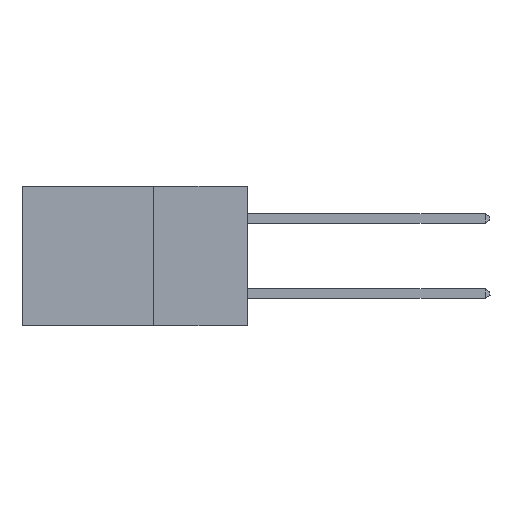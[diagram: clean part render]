
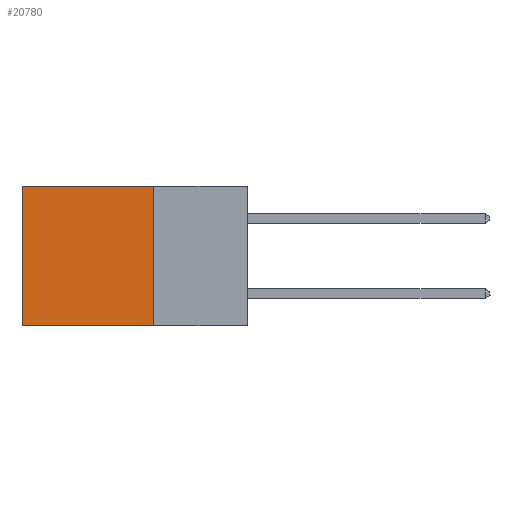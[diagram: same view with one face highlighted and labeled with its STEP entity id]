
A CAD part, left-side view. The second image highlights one B-rep face of the part: STEP entity #20780.
In plain terms, the highlighted planar face has unit normal (-1, 0, 0).
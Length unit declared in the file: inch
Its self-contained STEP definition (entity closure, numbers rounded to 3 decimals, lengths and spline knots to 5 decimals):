
#270 = VECTOR ( 'NONE', #4912, 39.37008 ) ;
#972 = CARTESIAN_POINT ( 'NONE',  ( 0.298, 0.25, 0. ) ) ;
#4577 = LINE ( 'NONE', #8691, #10844 ) ;
#4910 = CARTESIAN_POINT ( 'NONE',  ( 0.298, 0.6, -0.37 ) ) ;
#4912 = DIRECTION ( 'NONE',  ( 0., 0., -1. ) ) ;
#6288 = EDGE_CURVE ( 'NONE', #12097, #23439, #10033, .T. ) ;
#6700 = CARTESIAN_POINT ( 'NONE',  ( 0.298, 0.25, 0. ) ) ;
#6962 = DIRECTION ( 'NONE',  ( 1., 0., 0. ) ) ;
#7075 = PLANE ( 'NONE',  #17705 ) ;
#7313 = EDGE_LOOP ( 'NONE', ( #16508, #26935, #26849, #10260 ) ) ;
#7542 = DIRECTION ( 'NONE',  ( 0., 0., -1. ) ) ;
#7704 = VECTOR ( 'NONE', #7542, 39.37008 ) ;
#7769 = EDGE_CURVE ( 'NONE', #19668, #12097, #17508, .T. ) ;
#8394 = LINE ( 'NONE', #972, #7704 ) ;
#8691 = CARTESIAN_POINT ( 'NONE',  ( 0.298, 0.25, -0.37 ) ) ;
#9128 = CARTESIAN_POINT ( 'NONE',  ( 0.298, 0.6, 0. ) ) ;
#9564 = EDGE_CURVE ( 'NONE', #24120, #23439, #4577, .T. ) ;
#10033 = LINE ( 'NONE', #9128, #270 ) ;
#10260 = ORIENTED_EDGE ( 'NONE', *, *, #7769, .T. ) ;
#10844 = VECTOR ( 'NONE', #11333, 39.37008 ) ;
#10923 = DIRECTION ( 'NONE',  ( 0., 1., 0. ) ) ;
#11333 = DIRECTION ( 'NONE',  ( 0., 1., 0. ) ) ;
#12097 = VERTEX_POINT ( 'NONE', #16098 ) ;
#12647 = FACE_OUTER_BOUND ( 'NONE', #7313, .T. ) ;
#13826 = CARTESIAN_POINT ( 'NONE',  ( 0.298, 0.25, -0.37 ) ) ;
#16098 = CARTESIAN_POINT ( 'NONE',  ( 0.298, 0.6, 0. ) ) ;
#16508 = ORIENTED_EDGE ( 'NONE', *, *, #6288, .T. ) ;
#17508 = LINE ( 'NONE', #6700, #18941 ) ;
#17705 = AXIS2_PLACEMENT_3D ( 'NONE', #22172, #6962, #24603 ) ;
#18691 = EDGE_CURVE ( 'NONE', #19668, #24120, #8394, .T. ) ;
#18941 = VECTOR ( 'NONE', #10923, 39.37008 ) ;
#19668 = VERTEX_POINT ( 'NONE', #21869 ) ;
#20780 = ADVANCED_FACE ( 'NONE', ( #12647 ), #7075, .F. ) ;
#21869 = CARTESIAN_POINT ( 'NONE',  ( 0.298, 0.25, 0. ) ) ;
#22172 = CARTESIAN_POINT ( 'NONE',  ( 0.298, 0.25, 0. ) ) ;
#23439 = VERTEX_POINT ( 'NONE', #4910 ) ;
#24120 = VERTEX_POINT ( 'NONE', #13826 ) ;
#24603 = DIRECTION ( 'NONE',  ( 0., 0., -1. ) ) ;
#26849 = ORIENTED_EDGE ( 'NONE', *, *, #18691, .F. ) ;
#26935 = ORIENTED_EDGE ( 'NONE', *, *, #9564, .F. ) ;
